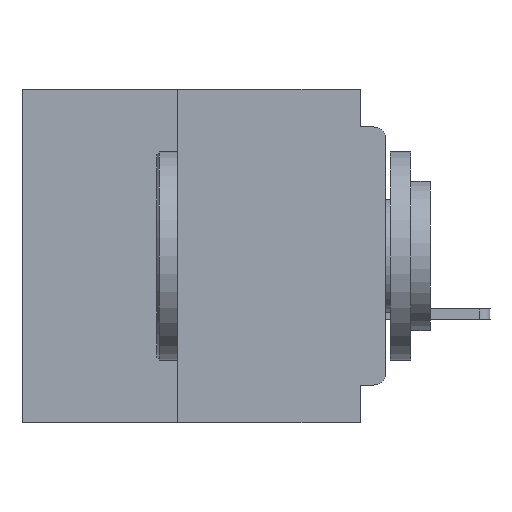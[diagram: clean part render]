
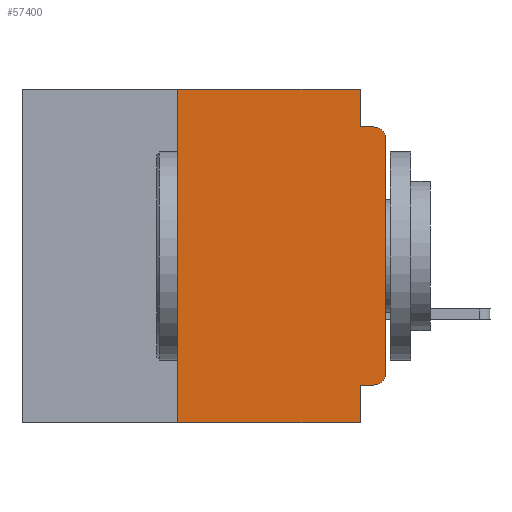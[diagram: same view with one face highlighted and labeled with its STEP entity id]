
A CAD part, left-side view. The second image highlights one B-rep face of the part: STEP entity #57400.
In plain terms, the highlighted planar face has unit normal (-1, 0, 0).
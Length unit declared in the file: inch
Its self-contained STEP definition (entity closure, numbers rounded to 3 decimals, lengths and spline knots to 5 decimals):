
#205 = ORIENTED_EDGE ( 'NONE', *, *, #24829, .F. ) ;
#861 = CARTESIAN_POINT ( 'NONE',  ( 0., 0.437, -0.4 ) ) ;
#1020 = VERTEX_POINT ( 'NONE', #51354 ) ;
#2001 = CARTESIAN_POINT ( 'NONE',  ( 0., 0.015, -0.34 ) ) ;
#2390 = VERTEX_POINT ( 'NONE', #54687 ) ;
#2757 = DIRECTION ( 'NONE',  ( 0., 0., -1. ) ) ;
#3187 = ORIENTED_EDGE ( 'NONE', *, *, #7771, .F. ) ;
#3529 = DIRECTION ( 'NONE',  ( 0., 0., -1. ) ) ;
#4672 = DIRECTION ( 'NONE',  ( 0., 0., 1. ) ) ;
#5330 = CARTESIAN_POINT ( 'NONE',  ( 0., 0.25, 0. ) ) ;
#6435 = VERTEX_POINT ( 'NONE', #20858 ) ;
#6783 = DIRECTION ( 'NONE',  ( 0., 0., -1. ) ) ;
#7771 = EDGE_CURVE ( 'NONE', #19161, #1020, #14004, .T. ) ;
#7779 = CARTESIAN_POINT ( 'NONE',  ( 0., 0., -0.06 ) ) ;
#9364 = ORIENTED_EDGE ( 'NONE', *, *, #29311, .T. ) ;
#10227 = EDGE_CURVE ( 'NONE', #48360, #2390, #57879, .T. ) ;
#11429 = VECTOR ( 'NONE', #49575, 39.37008 ) ;
#13488 = VECTOR ( 'NONE', #4672, 39.37008 ) ;
#14004 = LINE ( 'NONE', #54111, #26505 ) ;
#16289 = ORIENTED_EDGE ( 'NONE', *, *, #48527, .T. ) ;
#16709 = CIRCLE ( 'NONE', #32361, 0.015 ) ;
#17125 = ORIENTED_EDGE ( 'NONE', *, *, #21119, .T. ) ;
#17375 = FACE_OUTER_BOUND ( 'NONE', #27585, .T. ) ;
#18014 = EDGE_CURVE ( 'NONE', #58969, #44194, #33683, .T. ) ;
#18116 = AXIS2_PLACEMENT_3D ( 'NONE', #50423, #31731, #3529 ) ;
#19161 = VERTEX_POINT ( 'NONE', #60413 ) ;
#19353 = CARTESIAN_POINT ( 'NONE',  ( 0., 0., -0.045 ) ) ;
#20372 = AXIS2_PLACEMENT_3D ( 'NONE', #52406, #24228, #57123 ) ;
#20385 = VECTOR ( 'NONE', #56479, 39.37008 ) ;
#20858 = CARTESIAN_POINT ( 'NONE',  ( 0., 0.015, -0.045 ) ) ;
#21119 = EDGE_CURVE ( 'NONE', #34182, #6435, #25765, .T. ) ;
#22043 = VERTEX_POINT ( 'NONE', #40145 ) ;
#23294 = VERTEX_POINT ( 'NONE', #54372 ) ;
#24228 = DIRECTION ( 'NONE',  ( -1., 0., 0. ) ) ;
#24330 = ORIENTED_EDGE ( 'NONE', *, *, #37559, .F. ) ;
#24829 = EDGE_CURVE ( 'NONE', #1020, #44194, #56754, .T. ) ;
#25765 = CIRCLE ( 'NONE', #20372, 0.015 ) ;
#25960 = DIRECTION ( 'NONE',  ( 0., 1., 0. ) ) ;
#26226 = CARTESIAN_POINT ( 'NONE',  ( 0., 0.031, -0.4 ) ) ;
#26505 = VECTOR ( 'NONE', #25960, 39.37008 ) ;
#27585 = EDGE_LOOP ( 'NONE', ( #9364, #17125, #39926, #44894, #52639, #24330, #38511, #205, #3187, #16289 ) ) ;
#29311 = EDGE_CURVE ( 'NONE', #23294, #34182, #29471, .T. ) ;
#29471 = LINE ( 'NONE', #60277, #54470 ) ;
#31731 = DIRECTION ( 'NONE',  ( 1., 0., 0. ) ) ;
#32167 = DIRECTION ( 'NONE',  ( 0., 0., 1. ) ) ;
#32361 = AXIS2_PLACEMENT_3D ( 'NONE', #2001, #34951, #6783 ) ;
#33683 = LINE ( 'NONE', #861, #58641 ) ;
#33801 = DIRECTION ( 'NONE',  ( 0., -1., 0. ) ) ;
#34182 = VERTEX_POINT ( 'NONE', #7779 ) ;
#34951 = DIRECTION ( 'NONE',  ( -1., 0., 0. ) ) ;
#37559 = EDGE_CURVE ( 'NONE', #58969, #48360, #39966, .T. ) ;
#37908 = LINE ( 'NONE', #43625, #11429 ) ;
#38511 = ORIENTED_EDGE ( 'NONE', *, *, #18014, .T. ) ;
#39926 = ORIENTED_EDGE ( 'NONE', *, *, #46597, .F. ) ;
#39966 = LINE ( 'NONE', #51765, #13488 ) ;
#40145 = CARTESIAN_POINT ( 'NONE',  ( 0., 0.031, -0.045 ) ) ;
#42492 = CARTESIAN_POINT ( 'NONE',  ( 0., 0.437, 0. ) ) ;
#43072 = CARTESIAN_POINT ( 'NONE',  ( 0., 0.25, -0.4 ) ) ;
#43625 = CARTESIAN_POINT ( 'NONE',  ( 0., 0.031, 0. ) ) ;
#44194 = VERTEX_POINT ( 'NONE', #57023 ) ;
#44894 = ORIENTED_EDGE ( 'NONE', *, *, #57906, .F. ) ;
#45704 = PLANE ( 'NONE',  #18116 ) ;
#46597 = EDGE_CURVE ( 'NONE', #22043, #6435, #58993, .T. ) ;
#47498 = DIRECTION ( 'NONE',  ( 0., -1., 0. ) ) ;
#47976 = VECTOR ( 'NONE', #47498, 39.37008 ) ;
#48360 = VERTEX_POINT ( 'NONE', #5330 ) ;
#48527 = EDGE_CURVE ( 'NONE', #19161, #23294, #16709, .T. ) ;
#49575 = DIRECTION ( 'NONE',  ( 0., 0., -1. ) ) ;
#50423 = CARTESIAN_POINT ( 'NONE',  ( 0., 0.437, 0. ) ) ;
#51354 = CARTESIAN_POINT ( 'NONE',  ( 0., 0.031, -0.355 ) ) ;
#51765 = CARTESIAN_POINT ( 'NONE',  ( 0., 0.25, -0.4 ) ) ;
#52406 = CARTESIAN_POINT ( 'NONE',  ( 0., 0.015, -0.06 ) ) ;
#52639 = ORIENTED_EDGE ( 'NONE', *, *, #10227, .F. ) ;
#53811 = VECTOR ( 'NONE', #2757, 39.37008 ) ;
#54111 = CARTESIAN_POINT ( 'NONE',  ( 0., 0., -0.355 ) ) ;
#54372 = CARTESIAN_POINT ( 'NONE',  ( 0., 0., -0.34 ) ) ;
#54470 = VECTOR ( 'NONE', #32167, 39.37008 ) ;
#54687 = CARTESIAN_POINT ( 'NONE',  ( 0., 0.031, 0. ) ) ;
#56479 = DIRECTION ( 'NONE',  ( 0., -1., 0. ) ) ;
#56754 = LINE ( 'NONE', #26226, #53811 ) ;
#57023 = CARTESIAN_POINT ( 'NONE',  ( 0., 0.031, -0.4 ) ) ;
#57123 = DIRECTION ( 'NONE',  ( 0., 0., -1. ) ) ;
#57400 = ADVANCED_FACE ( 'NONE', ( #17375 ), #45704, .F. ) ;
#57879 = LINE ( 'NONE', #42492, #20385 ) ;
#57906 = EDGE_CURVE ( 'NONE', #2390, #22043, #37908, .T. ) ;
#58641 = VECTOR ( 'NONE', #33801, 39.37008 ) ;
#58969 = VERTEX_POINT ( 'NONE', #43072 ) ;
#58993 = LINE ( 'NONE', #19353, #47976 ) ;
#60277 = CARTESIAN_POINT ( 'NONE',  ( 0., 0., 0. ) ) ;
#60413 = CARTESIAN_POINT ( 'NONE',  ( 0., 0.015, -0.355 ) ) ;
